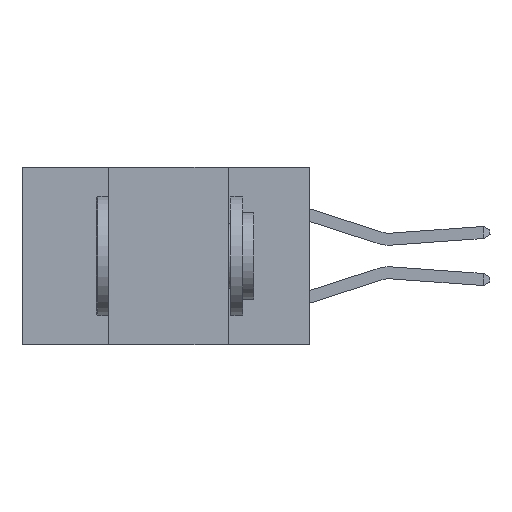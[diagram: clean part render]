
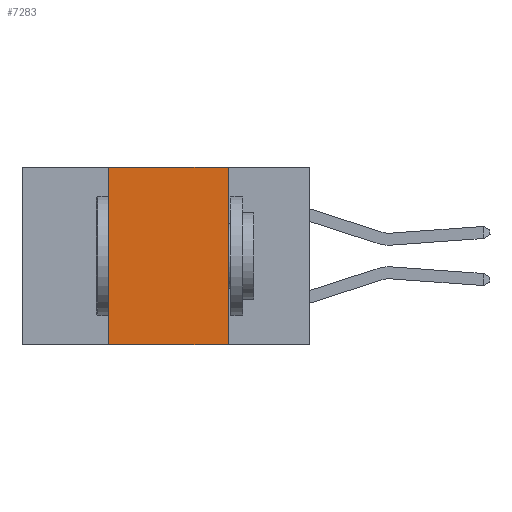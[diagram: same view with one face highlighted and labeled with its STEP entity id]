
A CAD part, left-side view. The second image highlights one B-rep face of the part: STEP entity #7283.
In plain terms, the highlighted planar face has unit normal (-1, 0, 0).
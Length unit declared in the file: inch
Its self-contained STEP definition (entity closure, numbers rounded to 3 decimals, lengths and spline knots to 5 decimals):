
#288 = DIRECTION ( 'NONE',  ( 1., 0., 0. ) ) ;
#1407 = EDGE_CURVE ( 'NONE', #18182, #13755, #13945, .T. ) ;
#2018 = EDGE_CURVE ( 'NONE', #13755, #12222, #5698, .T. ) ;
#2239 = LINE ( 'NONE', #2323, #3288 ) ;
#2323 = CARTESIAN_POINT ( 'NONE',  ( 0., 0.42, -0.37 ) ) ;
#2700 = CARTESIAN_POINT ( 'NONE',  ( 0., 0.6, -0.37 ) ) ;
#3288 = VECTOR ( 'NONE', #8074, 39.37008 ) ;
#3417 = ORIENTED_EDGE ( 'NONE', *, *, #5179, .T. ) ;
#4302 = DIRECTION ( 'NONE',  ( 0., -1., 0. ) ) ;
#4529 = VECTOR ( 'NONE', #16180, 39.37008 ) ;
#5179 = EDGE_CURVE ( 'NONE', #7365, #12222, #17347, .T. ) ;
#5698 = LINE ( 'NONE', #17240, #4529 ) ;
#5767 = PLANE ( 'NONE',  #13793 ) ;
#5958 = DIRECTION ( 'NONE',  ( 0., 0., -1. ) ) ;
#6424 = ORIENTED_EDGE ( 'NONE', *, *, #10728, .F. ) ;
#7283 = ADVANCED_FACE ( 'NONE', ( #15884 ), #5767, .F. ) ;
#7365 = VERTEX_POINT ( 'NONE', #7467 ) ;
#7467 = CARTESIAN_POINT ( 'NONE',  ( 0., 0.42, -0.37 ) ) ;
#8074 = DIRECTION ( 'NONE',  ( 0., 0., 1. ) ) ;
#8187 = DIRECTION ( 'NONE',  ( 0., -1., 0. ) ) ;
#10260 = CARTESIAN_POINT ( 'NONE',  ( 0., 0.17, -0.37 ) ) ;
#10503 = CARTESIAN_POINT ( 'NONE',  ( 0., 0.42, 0. ) ) ;
#10725 = EDGE_LOOP ( 'NONE', ( #11024, #16103, #6424, #3417 ) ) ;
#10728 = EDGE_CURVE ( 'NONE', #7365, #18182, #2239, .T. ) ;
#11024 = ORIENTED_EDGE ( 'NONE', *, *, #2018, .F. ) ;
#12036 = CARTESIAN_POINT ( 'NONE',  ( 0., 0.17, 0. ) ) ;
#12222 = VERTEX_POINT ( 'NONE', #10260 ) ;
#12886 = CARTESIAN_POINT ( 'NONE',  ( 0., 0.6, 0. ) ) ;
#13130 = CARTESIAN_POINT ( 'NONE',  ( 0., 0.6, 0. ) ) ;
#13755 = VERTEX_POINT ( 'NONE', #12036 ) ;
#13793 = AXIS2_PLACEMENT_3D ( 'NONE', #13130, #288, #5958 ) ;
#13945 = LINE ( 'NONE', #12886, #17298 ) ;
#14855 = VECTOR ( 'NONE', #4302, 39.37008 ) ;
#15884 = FACE_OUTER_BOUND ( 'NONE', #10725, .T. ) ;
#16103 = ORIENTED_EDGE ( 'NONE', *, *, #1407, .F. ) ;
#16180 = DIRECTION ( 'NONE',  ( 0., 0., -1. ) ) ;
#17240 = CARTESIAN_POINT ( 'NONE',  ( 0., 0.17, -0.37 ) ) ;
#17298 = VECTOR ( 'NONE', #8187, 39.37008 ) ;
#17347 = LINE ( 'NONE', #2700, #14855 ) ;
#18182 = VERTEX_POINT ( 'NONE', #10503 ) ;
